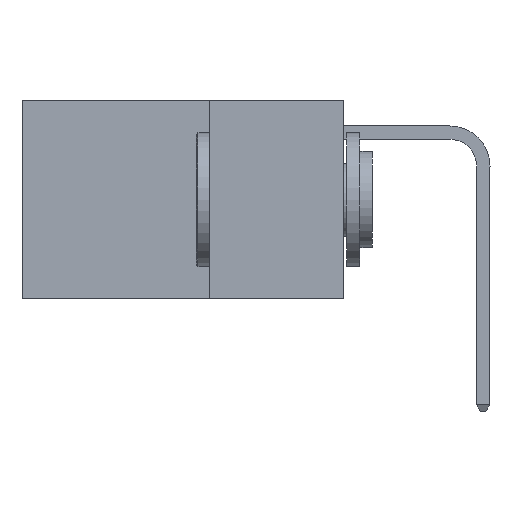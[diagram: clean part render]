
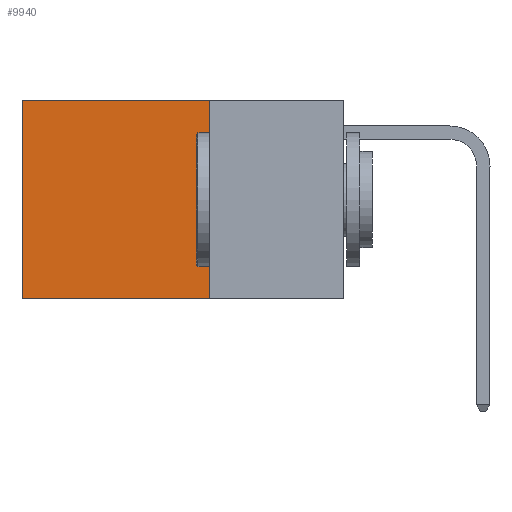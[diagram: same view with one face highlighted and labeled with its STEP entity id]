
A CAD part, left-side view. The second image highlights one B-rep face of the part: STEP entity #9940.
In plain terms, the highlighted planar face has unit normal (-1, 0, 0).
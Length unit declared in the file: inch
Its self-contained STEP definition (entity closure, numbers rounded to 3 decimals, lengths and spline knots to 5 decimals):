
#24 = EDGE_CURVE ( 'NONE', #3121, #4487, #10990, .T. ) ;
#1210 = CARTESIAN_POINT ( 'NONE',  ( 0.2625, 0.25, -0.37 ) ) ;
#1805 = LINE ( 'NONE', #14078, #13817 ) ;
#3067 = EDGE_CURVE ( 'NONE', #4487, #9945, #3598, .T. ) ;
#3121 = VERTEX_POINT ( 'NONE', #12623 ) ;
#3413 = DIRECTION ( 'NONE',  ( 0., 0., -1. ) ) ;
#3539 = VECTOR ( 'NONE', #3413, 39.37008 ) ;
#3598 = LINE ( 'NONE', #4701, #3539 ) ;
#4097 = FACE_OUTER_BOUND ( 'NONE', #14940, .T. ) ;
#4177 = ORIENTED_EDGE ( 'NONE', *, *, #3067, .T. ) ;
#4487 = VERTEX_POINT ( 'NONE', #7928 ) ;
#4701 = CARTESIAN_POINT ( 'NONE',  ( 0.2625, 0.6, 0. ) ) ;
#5336 = EDGE_CURVE ( 'NONE', #3121, #11657, #14868, .T. ) ;
#6233 = CARTESIAN_POINT ( 'NONE',  ( 0.2625, 0.6, -0.37 ) ) ;
#7200 = ORIENTED_EDGE ( 'NONE', *, *, #13259, .F. ) ;
#7645 = AXIS2_PLACEMENT_3D ( 'NONE', #8109, #8623, #10292 ) ;
#7928 = CARTESIAN_POINT ( 'NONE',  ( 0.2625, 0.6, 0. ) ) ;
#8109 = CARTESIAN_POINT ( 'NONE',  ( 0.2625, 0.25, 0. ) ) ;
#8143 = ORIENTED_EDGE ( 'NONE', *, *, #24, .T. ) ;
#8323 = PLANE ( 'NONE',  #7645 ) ;
#8623 = DIRECTION ( 'NONE',  ( 1., 0., 0. ) ) ;
#9940 = ADVANCED_FACE ( 'NONE', ( #4097 ), #8323, .F. ) ;
#9945 = VERTEX_POINT ( 'NONE', #6233 ) ;
#10292 = DIRECTION ( 'NONE',  ( 0., 0., -1. ) ) ;
#10751 = DIRECTION ( 'NONE',  ( 0., 0., -1. ) ) ;
#10819 = CARTESIAN_POINT ( 'NONE',  ( 0.2625, 0.25, 0. ) ) ;
#10903 = VECTOR ( 'NONE', #11384, 39.37008 ) ;
#10990 = LINE ( 'NONE', #12305, #10903 ) ;
#11384 = DIRECTION ( 'NONE',  ( 0., 1., 0. ) ) ;
#11657 = VERTEX_POINT ( 'NONE', #1210 ) ;
#11951 = DIRECTION ( 'NONE',  ( 0., 1., 0. ) ) ;
#12305 = CARTESIAN_POINT ( 'NONE',  ( 0.2625, 0.25, 0. ) ) ;
#12623 = CARTESIAN_POINT ( 'NONE',  ( 0.2625, 0.25, 0. ) ) ;
#13259 = EDGE_CURVE ( 'NONE', #11657, #9945, #1805, .T. ) ;
#13768 = ORIENTED_EDGE ( 'NONE', *, *, #5336, .F. ) ;
#13817 = VECTOR ( 'NONE', #11951, 39.37008 ) ;
#14078 = CARTESIAN_POINT ( 'NONE',  ( 0.2625, 0.25, -0.37 ) ) ;
#14858 = VECTOR ( 'NONE', #10751, 39.37008 ) ;
#14868 = LINE ( 'NONE', #10819, #14858 ) ;
#14940 = EDGE_LOOP ( 'NONE', ( #4177, #7200, #13768, #8143 ) ) ;
